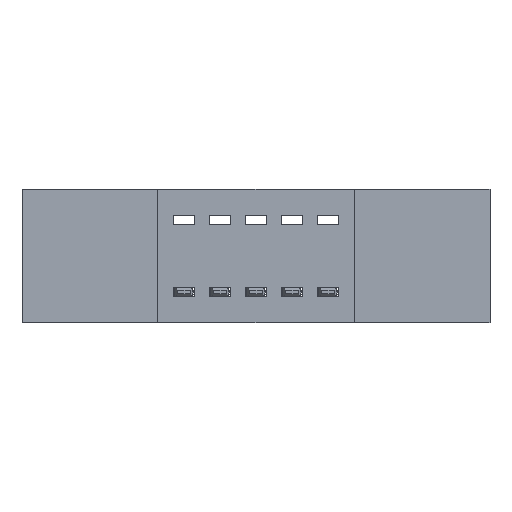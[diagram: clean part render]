
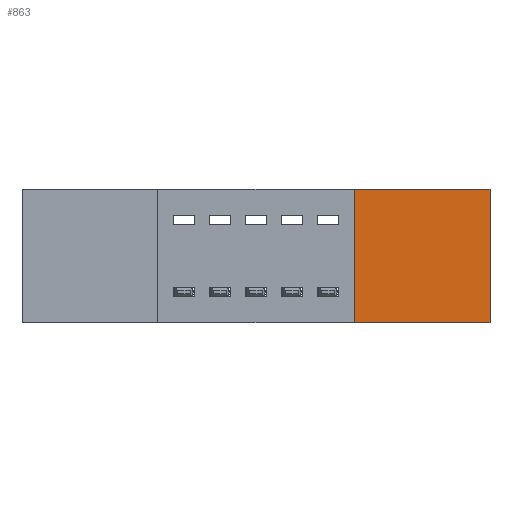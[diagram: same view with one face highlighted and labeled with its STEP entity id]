
A CAD part, front view. The second image highlights one B-rep face of the part: STEP entity #863.
In plain terms, the highlighted planar face has unit normal (0, -1, 0).
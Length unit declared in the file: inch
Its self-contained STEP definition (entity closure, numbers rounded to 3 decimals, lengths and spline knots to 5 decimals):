
#373 = CARTESIAN_POINT ( 'NONE',  ( 0.923, 0., 0. ) ) ;
#480 = FACE_OUTER_BOUND ( 'NONE', #7032, .T. ) ;
#735 = VECTOR ( 'NONE', #7314, 39.37008 ) ;
#863 = ADVANCED_FACE ( 'NONE', ( #480 ), #5555, .T. ) ;
#1009 = EDGE_CURVE ( 'NONE', #7324, #1887, #5629, .T. ) ;
#1287 = VECTOR ( 'NONE', #2813, 39.37008 ) ;
#1410 = DIRECTION ( 'NONE',  ( 1., 0., 0. ) ) ;
#1723 = EDGE_CURVE ( 'NONE', #2212, #6602, #7227, .T. ) ;
#1772 = CARTESIAN_POINT ( 'NONE',  ( 1.3, 0., 0. ) ) ;
#1857 = ORIENTED_EDGE ( 'NONE', *, *, #1723, .F. ) ;
#1887 = VERTEX_POINT ( 'NONE', #4107 ) ;
#1942 = CARTESIAN_POINT ( 'NONE',  ( 0., 0., 0. ) ) ;
#2212 = VERTEX_POINT ( 'NONE', #373 ) ;
#2527 = VECTOR ( 'NONE', #4182, 39.37008 ) ;
#2813 = DIRECTION ( 'NONE',  ( 0., 0., 1. ) ) ;
#3221 = VECTOR ( 'NONE', #1410, 39.37008 ) ;
#3250 = LINE ( 'NONE', #3420, #1287 ) ;
#3420 = CARTESIAN_POINT ( 'NONE',  ( 0.923, 0., -0.37 ) ) ;
#4107 = CARTESIAN_POINT ( 'NONE',  ( 0.923, 0., -0.37 ) ) ;
#4182 = DIRECTION ( 'NONE',  ( -1., 0., 0. ) ) ;
#4265 = LINE ( 'NONE', #7104, #735 ) ;
#4412 = ORIENTED_EDGE ( 'NONE', *, *, #6236, .F. ) ;
#4938 = ORIENTED_EDGE ( 'NONE', *, *, #6614, .F. ) ;
#4960 = ORIENTED_EDGE ( 'NONE', *, *, #1009, .F. ) ;
#5517 = CARTESIAN_POINT ( 'NONE',  ( 0., 0., -0.37 ) ) ;
#5548 = AXIS2_PLACEMENT_3D ( 'NONE', #5517, #5554, #5634 ) ;
#5554 = DIRECTION ( 'NONE',  ( 0., -1., 0. ) ) ;
#5555 = PLANE ( 'NONE',  #5548 ) ;
#5629 = LINE ( 'NONE', #6679, #2527 ) ;
#5634 = DIRECTION ( 'NONE',  ( 0., 0., -1. ) ) ;
#6236 = EDGE_CURVE ( 'NONE', #6602, #7324, #4265, .T. ) ;
#6352 = CARTESIAN_POINT ( 'NONE',  ( 1.3, 0., -0.37 ) ) ;
#6602 = VERTEX_POINT ( 'NONE', #1772 ) ;
#6614 = EDGE_CURVE ( 'NONE', #1887, #2212, #3250, .T. ) ;
#6679 = CARTESIAN_POINT ( 'NONE',  ( 0., 0., -0.37 ) ) ;
#7032 = EDGE_LOOP ( 'NONE', ( #4938, #4960, #4412, #1857 ) ) ;
#7104 = CARTESIAN_POINT ( 'NONE',  ( 1.3, 0., 0. ) ) ;
#7227 = LINE ( 'NONE', #1942, #3221 ) ;
#7314 = DIRECTION ( 'NONE',  ( 0., 0., -1. ) ) ;
#7324 = VERTEX_POINT ( 'NONE', #6352 ) ;
